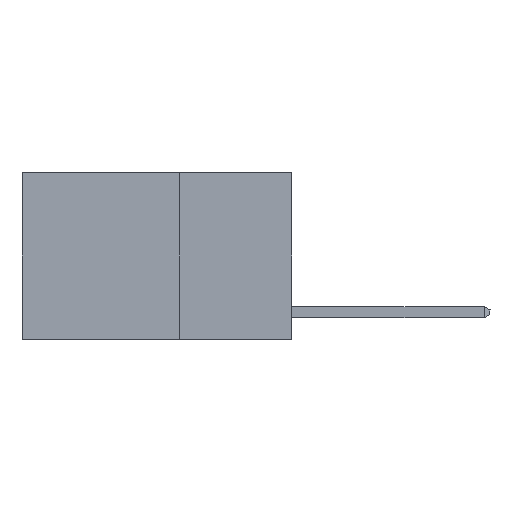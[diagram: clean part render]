
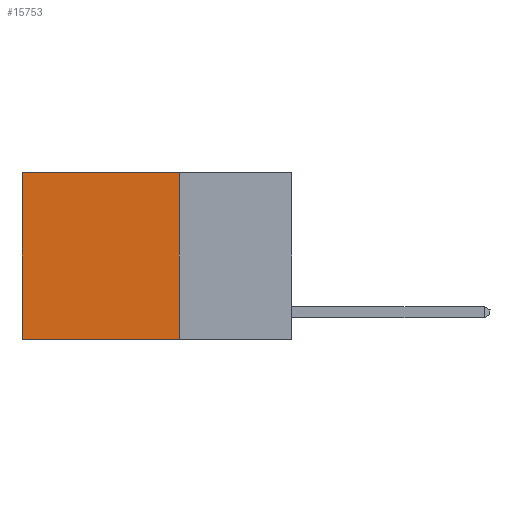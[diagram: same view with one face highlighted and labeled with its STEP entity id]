
A CAD part, left-side view. The second image highlights one B-rep face of the part: STEP entity #15753.
In plain terms, the highlighted planar face has unit normal (-1, 0, 0).
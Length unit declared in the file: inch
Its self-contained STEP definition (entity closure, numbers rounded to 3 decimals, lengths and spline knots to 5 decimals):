
#321 = VERTEX_POINT ( 'NONE', #5860 ) ;
#489 = VERTEX_POINT ( 'NONE', #2651 ) ;
#672 = EDGE_CURVE ( 'NONE', #321, #489, #16169, .T. ) ;
#756 = DIRECTION ( 'NONE',  ( 1., 0., 0. ) ) ;
#1331 = EDGE_CURVE ( 'NONE', #7339, #489, #15550, .T. ) ;
#2651 = CARTESIAN_POINT ( 'NONE',  ( 0.2625, 0.6, -0.37 ) ) ;
#2761 = VECTOR ( 'NONE', #8438, 39.37008 ) ;
#3076 = LINE ( 'NONE', #11735, #16131 ) ;
#3894 = VECTOR ( 'NONE', #11015, 39.37008 ) ;
#4636 = CARTESIAN_POINT ( 'NONE',  ( 0.2625, 0.25, -0.37 ) ) ;
#5756 = FACE_OUTER_BOUND ( 'NONE', #11825, .T. ) ;
#5843 = CARTESIAN_POINT ( 'NONE',  ( 0.2625, 0.25, 0. ) ) ;
#5860 = CARTESIAN_POINT ( 'NONE',  ( 0.2625, 0.6, 0. ) ) ;
#6121 = LINE ( 'NONE', #9809, #2761 ) ;
#6624 = DIRECTION ( 'NONE',  ( 0., 0., -1. ) ) ;
#7303 = VECTOR ( 'NONE', #6624, 39.37008 ) ;
#7339 = VERTEX_POINT ( 'NONE', #10043 ) ;
#7624 = ORIENTED_EDGE ( 'NONE', *, *, #8615, .T. ) ;
#8275 = ORIENTED_EDGE ( 'NONE', *, *, #16227, .F. ) ;
#8438 = DIRECTION ( 'NONE',  ( 0., 0., -1. ) ) ;
#8615 = EDGE_CURVE ( 'NONE', #9201, #321, #3076, .T. ) ;
#9134 = DIRECTION ( 'NONE',  ( 0., 1., 0. ) ) ;
#9201 = VERTEX_POINT ( 'NONE', #13663 ) ;
#9563 = PLANE ( 'NONE',  #11262 ) ;
#9611 = DIRECTION ( 'NONE',  ( 0., 0., -1. ) ) ;
#9809 = CARTESIAN_POINT ( 'NONE',  ( 0.2625, 0.25, 0. ) ) ;
#10043 = CARTESIAN_POINT ( 'NONE',  ( 0.2625, 0.25, -0.37 ) ) ;
#11015 = DIRECTION ( 'NONE',  ( 0., 1., 0. ) ) ;
#11262 = AXIS2_PLACEMENT_3D ( 'NONE', #5843, #756, #9611 ) ;
#11735 = CARTESIAN_POINT ( 'NONE',  ( 0.2625, 0.25, 0. ) ) ;
#11825 = EDGE_LOOP ( 'NONE', ( #13898, #14101, #8275, #7624 ) ) ;
#13663 = CARTESIAN_POINT ( 'NONE',  ( 0.2625, 0.25, 0. ) ) ;
#13898 = ORIENTED_EDGE ( 'NONE', *, *, #672, .T. ) ;
#14101 = ORIENTED_EDGE ( 'NONE', *, *, #1331, .F. ) ;
#15459 = CARTESIAN_POINT ( 'NONE',  ( 0.2625, 0.6, 0. ) ) ;
#15550 = LINE ( 'NONE', #4636, #3894 ) ;
#15753 = ADVANCED_FACE ( 'NONE', ( #5756 ), #9563, .F. ) ;
#16131 = VECTOR ( 'NONE', #9134, 39.37008 ) ;
#16169 = LINE ( 'NONE', #15459, #7303 ) ;
#16227 = EDGE_CURVE ( 'NONE', #9201, #7339, #6121, .T. ) ;
